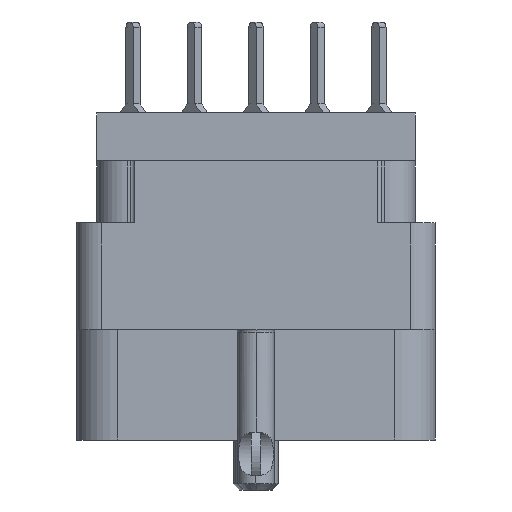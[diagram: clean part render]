
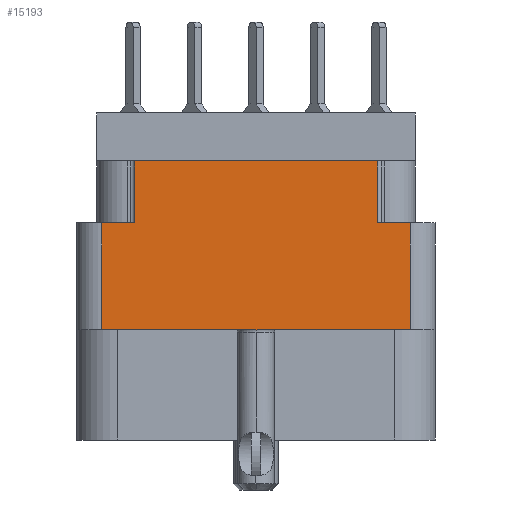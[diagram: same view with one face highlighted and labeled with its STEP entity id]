
A CAD part, left-side view. The second image highlights one B-rep face of the part: STEP entity #15193.
In plain terms, the highlighted planar face has unit normal (-1, 0, 0).
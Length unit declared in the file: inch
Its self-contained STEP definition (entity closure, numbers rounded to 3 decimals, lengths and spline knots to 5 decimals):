
#1004 = CARTESIAN_POINT ( 'NONE',  ( -1., 0.376, -0.798 ) ) ;
#1058 = ORIENTED_EDGE ( 'NONE', *, *, #45232, .F. ) ;
#1745 = DIRECTION ( 'NONE',  ( 0., 0., 1. ) ) ;
#1804 = CARTESIAN_POINT ( 'NONE',  ( -1., 0.376, -0.529 ) ) ;
#2199 = VERTEX_POINT ( 'NONE', #11561 ) ;
#3118 = LINE ( 'NONE', #20598, #15813 ) ;
#3141 = CARTESIAN_POINT ( 'NONE',  ( -1., -0.376, -0.798 ) ) ;
#3479 = EDGE_CURVE ( 'NONE', #26535, #9150, #35838, .T. ) ;
#3591 = ORIENTED_EDGE ( 'NONE', *, *, #3479, .F. ) ;
#3952 = DIRECTION ( 'NONE',  ( 0., -1., 0. ) ) ;
#4565 = ORIENTED_EDGE ( 'NONE', *, *, #37258, .T. ) ;
#4587 = FACE_OUTER_BOUND ( 'NONE', #8330, .T. ) ;
#6852 = VECTOR ( 'NONE', #3952, 39.37008 ) ;
#6907 = CARTESIAN_POINT ( 'NONE',  ( -1., 0.376, -0.268 ) ) ;
#7302 = LINE ( 'NONE', #14928, #14472 ) ;
#7615 = CARTESIAN_POINT ( 'NONE',  ( -1., -0.376, -0.529 ) ) ;
#8125 = VECTOR ( 'NONE', #1745, 39.37008 ) ;
#8330 = EDGE_LOOP ( 'NONE', ( #24458, #22547, #32688, #21373, #4565, #3591, #1058, #38724 ) ) ;
#8414 = VERTEX_POINT ( 'NONE', #1804 ) ;
#9150 = VERTEX_POINT ( 'NONE', #36098 ) ;
#9905 = DIRECTION ( 'NONE',  ( -1., 0., 0. ) ) ;
#11561 = CARTESIAN_POINT ( 'NONE',  ( -1., -0.376, -0.268 ) ) ;
#11780 = EDGE_CURVE ( 'NONE', #12627, #15218, #27243, .T. ) ;
#12627 = VERTEX_POINT ( 'NONE', #6907 ) ;
#13472 = DIRECTION ( 'NONE',  ( 0., 0., 1. ) ) ;
#14472 = VECTOR ( 'NONE', #22368, 39.37008 ) ;
#14904 = DIRECTION ( 'NONE',  ( 0., 0., 1. ) ) ;
#14928 = CARTESIAN_POINT ( 'NONE',  ( -1., -0.296, -0.268 ) ) ;
#15193 = ADVANCED_FACE ( 'NONE', ( #4587 ), #23859, .T. ) ;
#15218 = VERTEX_POINT ( 'NONE', #20580 ) ;
#15813 = VECTOR ( 'NONE', #31585, 39.37008 ) ;
#18680 = EDGE_CURVE ( 'NONE', #8414, #12627, #33076, .T. ) ;
#18863 = DIRECTION ( 'NONE',  ( 0., -1., 0. ) ) ;
#20580 = CARTESIAN_POINT ( 'NONE',  ( -1., 0.296, -0.268 ) ) ;
#20598 = CARTESIAN_POINT ( 'NONE',  ( -1., -0.376, -0.798 ) ) ;
#21373 = ORIENTED_EDGE ( 'NONE', *, *, #26919, .F. ) ;
#21435 = VECTOR ( 'NONE', #14904, 39.37008 ) ;
#22092 = VERTEX_POINT ( 'NONE', #30780 ) ;
#22368 = DIRECTION ( 'NONE',  ( 0., -1., 0. ) ) ;
#22547 = ORIENTED_EDGE ( 'NONE', *, *, #35481, .T. ) ;
#23859 = PLANE ( 'NONE',  #32935 ) ;
#24357 = EDGE_CURVE ( 'NONE', #44575, #2199, #3118, .T. ) ;
#24458 = ORIENTED_EDGE ( 'NONE', *, *, #18680, .F. ) ;
#25776 = CARTESIAN_POINT ( 'NONE',  ( -1., 0.296, -0.268 ) ) ;
#26535 = VERTEX_POINT ( 'NONE', #32026 ) ;
#26834 = LINE ( 'NONE', #33239, #44529 ) ;
#26919 = EDGE_CURVE ( 'NONE', #22092, #2199, #7302, .T. ) ;
#27243 = LINE ( 'NONE', #32540, #6852 ) ;
#30013 = CARTESIAN_POINT ( 'NONE',  ( -1., 0.438, -0.117 ) ) ;
#30780 = CARTESIAN_POINT ( 'NONE',  ( -1., -0.296, -0.268 ) ) ;
#31585 = DIRECTION ( 'NONE',  ( 0., 0., 1. ) ) ;
#32026 = CARTESIAN_POINT ( 'NONE',  ( -1., 0.296, -0.117 ) ) ;
#32540 = CARTESIAN_POINT ( 'NONE',  ( -1., 0.438, -0.268 ) ) ;
#32688 = ORIENTED_EDGE ( 'NONE', *, *, #24357, .T. ) ;
#32935 = AXIS2_PLACEMENT_3D ( 'NONE', #3141, #9905, #13472 ) ;
#33076 = LINE ( 'NONE', #1004, #21435 ) ;
#33239 = CARTESIAN_POINT ( 'NONE',  ( -1., 0., -0.529 ) ) ;
#33588 = LINE ( 'NONE', #25776, #41864 ) ;
#34127 = LINE ( 'NONE', #44077, #8125 ) ;
#35481 = EDGE_CURVE ( 'NONE', #8414, #44575, #26834, .T. ) ;
#35838 = LINE ( 'NONE', #30013, #41409 ) ;
#36098 = CARTESIAN_POINT ( 'NONE',  ( -1., -0.296, -0.117 ) ) ;
#37258 = EDGE_CURVE ( 'NONE', #22092, #9150, #34127, .T. ) ;
#38724 = ORIENTED_EDGE ( 'NONE', *, *, #11780, .F. ) ;
#39966 = DIRECTION ( 'NONE',  ( 0., 0., 1. ) ) ;
#41409 = VECTOR ( 'NONE', #44223, 39.37008 ) ;
#41864 = VECTOR ( 'NONE', #39966, 39.37008 ) ;
#44077 = CARTESIAN_POINT ( 'NONE',  ( -1., -0.296, -0.268 ) ) ;
#44223 = DIRECTION ( 'NONE',  ( 0., -1., 0. ) ) ;
#44529 = VECTOR ( 'NONE', #18863, 39.37008 ) ;
#44575 = VERTEX_POINT ( 'NONE', #7615 ) ;
#45232 = EDGE_CURVE ( 'NONE', #15218, #26535, #33588, .T. ) ;
